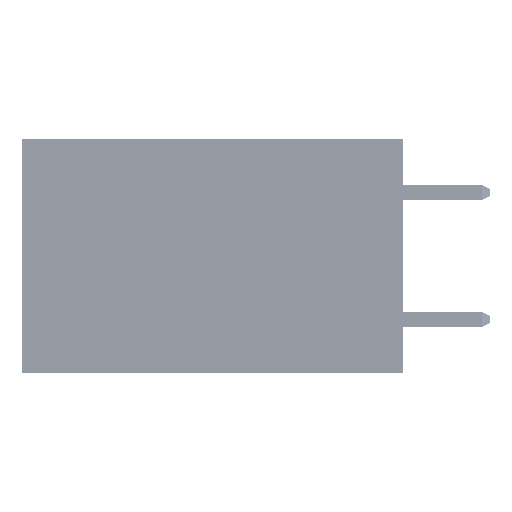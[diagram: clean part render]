
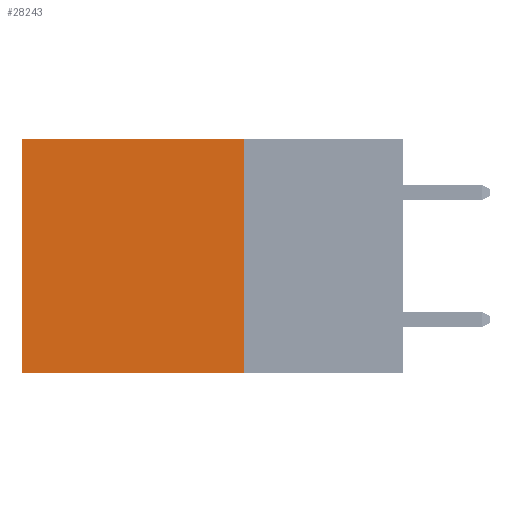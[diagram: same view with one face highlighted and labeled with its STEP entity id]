
A CAD part, left-side view. The second image highlights one B-rep face of the part: STEP entity #28243.
In plain terms, the highlighted planar face has unit normal (-1, 0, 0).
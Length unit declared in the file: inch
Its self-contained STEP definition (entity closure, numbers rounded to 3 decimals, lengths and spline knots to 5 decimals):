
#1004 = ORIENTED_EDGE ( 'NONE', *, *, #49346, .T. ) ;
#1441 = ORIENTED_EDGE ( 'NONE', *, *, #28165, .T. ) ;
#2935 = VECTOR ( 'NONE', #6284, 39.37008 ) ;
#4654 = DIRECTION ( 'NONE',  ( 0., 0., -1. ) ) ;
#6284 = DIRECTION ( 'NONE',  ( 0., 1., 0. ) ) ;
#6891 = ORIENTED_EDGE ( 'NONE', *, *, #43402, .F. ) ;
#9327 = CARTESIAN_POINT ( 'NONE',  ( 0.2875, 0.25, 0. ) ) ;
#10156 = LINE ( 'NONE', #36746, #49038 ) ;
#10361 = CARTESIAN_POINT ( 'NONE',  ( 0.2875, 0.25, 0. ) ) ;
#13106 = DIRECTION ( 'NONE',  ( 0., 0., -1. ) ) ;
#14573 = LINE ( 'NONE', #10361, #2935 ) ;
#17073 = ORIENTED_EDGE ( 'NONE', *, *, #33425, .F. ) ;
#20598 = FACE_OUTER_BOUND ( 'NONE', #28251, .T. ) ;
#21344 = VERTEX_POINT ( 'NONE', #44777 ) ;
#21703 = LINE ( 'NONE', #30846, #34710 ) ;
#26919 = VECTOR ( 'NONE', #4654, 39.37008 ) ;
#28165 = EDGE_CURVE ( 'NONE', #47238, #37662, #10156, .T. ) ;
#28243 = ADVANCED_FACE ( 'NONE', ( #20598 ), #32947, .F. ) ;
#28251 = EDGE_LOOP ( 'NONE', ( #1441, #17073, #6891, #1004 ) ) ;
#30846 = CARTESIAN_POINT ( 'NONE',  ( 0.2875, 0.25, -0.37 ) ) ;
#31700 = AXIS2_PLACEMENT_3D ( 'NONE', #9327, #36928, #44500 ) ;
#32947 = PLANE ( 'NONE',  #31700 ) ;
#33101 = VERTEX_POINT ( 'NONE', #33109 ) ;
#33109 = CARTESIAN_POINT ( 'NONE',  ( 0.2875, 0.25, -0.37 ) ) ;
#33425 = EDGE_CURVE ( 'NONE', #33101, #37662, #21703, .T. ) ;
#34710 = VECTOR ( 'NONE', #42241, 39.37008 ) ;
#35865 = CARTESIAN_POINT ( 'NONE',  ( 0.2875, 0.25, 0. ) ) ;
#36746 = CARTESIAN_POINT ( 'NONE',  ( 0.2875, 0.6, 0. ) ) ;
#36928 = DIRECTION ( 'NONE',  ( 1., 0., 0. ) ) ;
#37662 = VERTEX_POINT ( 'NONE', #43417 ) ;
#42241 = DIRECTION ( 'NONE',  ( 0., 1., 0. ) ) ;
#43402 = EDGE_CURVE ( 'NONE', #21344, #33101, #43593, .T. ) ;
#43417 = CARTESIAN_POINT ( 'NONE',  ( 0.2875, 0.6, -0.37 ) ) ;
#43593 = LINE ( 'NONE', #35865, #26919 ) ;
#44500 = DIRECTION ( 'NONE',  ( 0., 0., -1. ) ) ;
#44777 = CARTESIAN_POINT ( 'NONE',  ( 0.2875, 0.25, 0. ) ) ;
#45457 = CARTESIAN_POINT ( 'NONE',  ( 0.2875, 0.6, 0. ) ) ;
#47238 = VERTEX_POINT ( 'NONE', #45457 ) ;
#49038 = VECTOR ( 'NONE', #13106, 39.37008 ) ;
#49346 = EDGE_CURVE ( 'NONE', #21344, #47238, #14573, .T. ) ;
